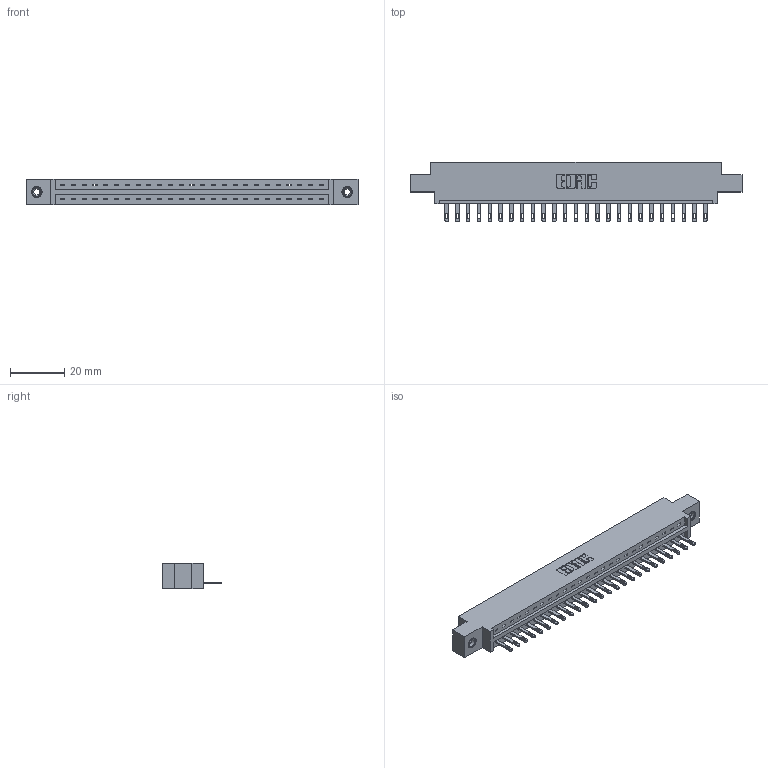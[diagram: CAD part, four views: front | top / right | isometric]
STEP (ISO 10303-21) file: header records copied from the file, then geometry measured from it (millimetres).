
FILE_DESCRIPTION (( 'STEP AP203' ), '1' );
FILE_NAME ('887-025-500-608.STEP', '2020-09-20T19:25:31', ( '' ), ( '' ), 'SwSTEP 2.0', 'SolidWorks 2020', '' );
FILE_SCHEMA (( 'CONFIG_CONTROL_DESIGN' ));
Length unit declared in the file: inch
Products named in the file (4): 345-250-001_345-250-003-102; 345-292-001_345-293-100; 837 Part_0.170 Offset - 0.156 Dia-TI; 887-025-500-608
Assembly tree (28 placements, depth 2):
  887-025-500-608
    837 Part_0.170 Offset - 0.156 Dia-TI
    345-292-001_345-293-100  x25
    345-250-001_345-250-003-102  x2
Bounding box: 122.07 x 21.85 x 9.4 mm (x, y, z)
Volume: 12366.1 mm3; surface area: 12868.7 mm2
Topology: 28 solids, 28 shells, 1628 faces, 4959 edges, 3298 vertices
Faces by surface type: plane 1106, cylinder 506, cone 12, torus 4
Entity records: 22030 total; most frequent: CARTESIAN_POINT 3816, ORIENTED_EDGE 3770, DIRECTION 3281, EDGE_CURVE 1885, VECTOR 1733, LINE 1733, VERTEX_POINT 1252, AXIS2_PLACEMENT_3D 774
